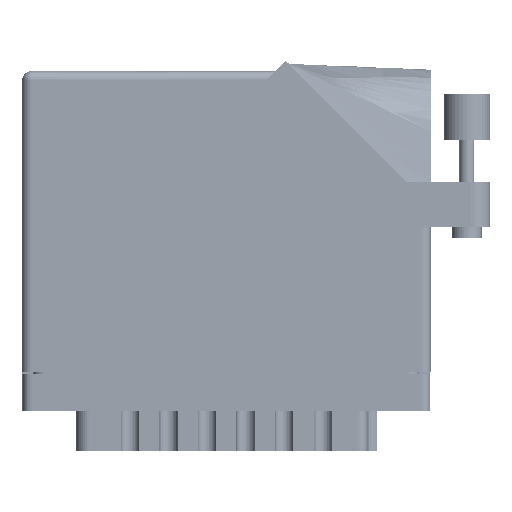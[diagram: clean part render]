
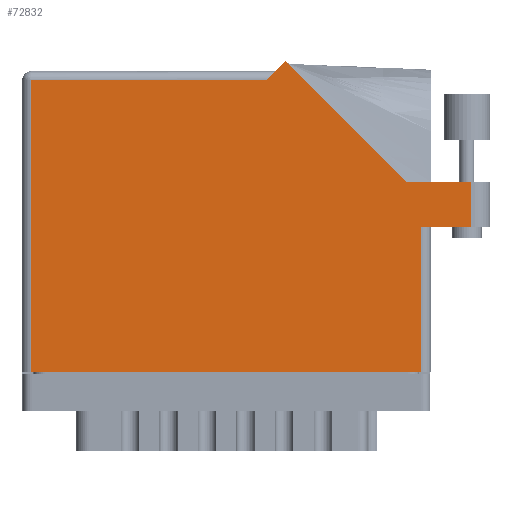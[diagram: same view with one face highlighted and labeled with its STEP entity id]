
A CAD part, front view. The second image highlights one B-rep face of the part: STEP entity #72832.
In plain terms, the highlighted face is planar.
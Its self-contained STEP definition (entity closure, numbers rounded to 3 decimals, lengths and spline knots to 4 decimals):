
#4905 = CARTESIAN_POINT ( 'NONE',  ( 0., 1.968, 0. ) ) ;
#5638 = CARTESIAN_POINT ( 'NONE',  ( 0., 2.03, 0. ) ) ;
#6931 = LINE ( 'NONE', #53528, #57470 ) ;
#7998 = EDGE_CURVE ( 'NONE', #71856, #78799, #75093, .T. ) ;
#9601 = VERTEX_POINT ( 'NONE', #84954 ) ;
#10204 = EDGE_CURVE ( 'NONE', #71552, #9601, #36644, .T. ) ;
#10798 = LINE ( 'NONE', #4905, #80476 ) ;
#12961 = CARTESIAN_POINT ( 'NONE',  ( 1.643, 1.968, 0. ) ) ;
#13494 = EDGE_LOOP ( 'NONE', ( #43923, #25591, #16066, #30915, #53617, #55203, #21313, #58799, #81192 ) ) ;
#13586 = CARTESIAN_POINT ( 'NONE',  ( 0., 0., 0. ) ) ;
#13745 = CARTESIAN_POINT ( 'NONE',  ( 3.155, 1.287, 0. ) ) ;
#14308 = DIRECTION ( 'NONE',  ( 1., 0., 0. ) ) ;
#14801 = VERTEX_POINT ( 'NONE', #86908 ) ;
#16066 = ORIENTED_EDGE ( 'NONE', *, *, #7998, .T. ) ;
#16969 = VECTOR ( 'NONE', #73017, 39.3701 ) ;
#19420 = DIRECTION ( 'NONE',  ( 0., 0., -1. ) ) ;
#21313 = ORIENTED_EDGE ( 'NONE', *, *, #48094, .T. ) ;
#22695 = DIRECTION ( 'NONE',  ( 1., 0., 0. ) ) ;
#22903 = DIRECTION ( 'NONE',  ( 0., 1., 0. ) ) ;
#23360 = CARTESIAN_POINT ( 'NONE',  ( 3.03, 1.287, 0. ) ) ;
#24436 = CARTESIAN_POINT ( 'NONE',  ( 0.062, 0., 0. ) ) ;
#25302 = VERTEX_POINT ( 'NONE', #70182 ) ;
#25591 = ORIENTED_EDGE ( 'NONE', *, *, #79175, .T. ) ;
#26758 = VECTOR ( 'NONE', #59239, 39.3701 ) ;
#30915 = ORIENTED_EDGE ( 'NONE', *, *, #80389, .T. ) ;
#31185 = DIRECTION ( 'NONE',  ( -0.707, 0.707, 0. ) ) ;
#34341 = VECTOR ( 'NONE', #22695, 39.3701 ) ;
#36644 = LINE ( 'NONE', #13586, #34341 ) ;
#38590 = DIRECTION ( 'NONE',  ( 0., -1., 0. ) ) ;
#43007 = VERTEX_POINT ( 'NONE', #84961 ) ;
#43923 = ORIENTED_EDGE ( 'NONE', *, *, #56450, .T. ) ;
#46718 = EDGE_CURVE ( 'NONE', #14801, #53883, #68690, .T. ) ;
#47881 = DIRECTION ( 'NONE',  ( -1., 0., 0. ) ) ;
#48024 = PLANE ( 'NONE',  #80949 ) ;
#48094 = EDGE_CURVE ( 'NONE', #43007, #71552, #80827, .T. ) ;
#49287 = VECTOR ( 'NONE', #72894, 39.3701 ) ;
#49854 = LINE ( 'NONE', #72097, #84590 ) ;
#50778 = VERTEX_POINT ( 'NONE', #72921 ) ;
#53528 = CARTESIAN_POINT ( 'NONE',  ( 2.5894, 1.287, 0. ) ) ;
#53617 = ORIENTED_EDGE ( 'NONE', *, *, #46718, .T. ) ;
#53883 = VERTEX_POINT ( 'NONE', #12961 ) ;
#55203 = ORIENTED_EDGE ( 'NONE', *, *, #65102, .T. ) ;
#56450 = EDGE_CURVE ( 'NONE', #25302, #50778, #49854, .T. ) ;
#57470 = VECTOR ( 'NONE', #31185, 39.3701 ) ;
#58799 = ORIENTED_EDGE ( 'NONE', *, *, #10204, .T. ) ;
#59239 = DIRECTION ( 'NONE',  ( -1., 0., 0. ) ) ;
#61602 = LINE ( 'NONE', #86400, #49287 ) ;
#62730 = DIRECTION ( 'NONE',  ( -1., 0., 0. ) ) ;
#65099 = CARTESIAN_POINT ( 'NONE',  ( 0.062, 0., 0. ) ) ;
#65102 = EDGE_CURVE ( 'NONE', #53883, #43007, #10798, .T. ) ;
#68690 = LINE ( 'NONE', #72099, #16969 ) ;
#70182 = CARTESIAN_POINT ( 'NONE',  ( 2.693, 0.98, 0. ) ) ;
#71552 = VERTEX_POINT ( 'NONE', #65099 ) ;
#71856 = VERTEX_POINT ( 'NONE', #23360 ) ;
#72097 = CARTESIAN_POINT ( 'NONE',  ( 2.755, 0.98, 0. ) ) ;
#72099 = CARTESIAN_POINT ( 'NONE',  ( 1.705, 2.03, 0. ) ) ;
#72832 = ADVANCED_FACE ( 'NONE', ( #77799 ), #48024, .F. ) ;
#72842 = LINE ( 'NONE', #80706, #89682 ) ;
#72894 = DIRECTION ( 'NONE',  ( 0., 1., 0. ) ) ;
#72921 = CARTESIAN_POINT ( 'NONE',  ( 3.03, 0.98, 0. ) ) ;
#73017 = DIRECTION ( 'NONE',  ( -0.707, -0.707, 0. ) ) ;
#75093 = LINE ( 'NONE', #13745, #26758 ) ;
#76972 = CARTESIAN_POINT ( 'NONE',  ( 2.5894, 1.287, 0. ) ) ;
#77799 = FACE_OUTER_BOUND ( 'NONE', #13494, .T. ) ;
#78799 = VERTEX_POINT ( 'NONE', #76972 ) ;
#79175 = EDGE_CURVE ( 'NONE', #50778, #71856, #72842, .T. ) ;
#80389 = EDGE_CURVE ( 'NONE', #78799, #14801, #6931, .T. ) ;
#80476 = VECTOR ( 'NONE', #47881, 39.3701 ) ;
#80706 = CARTESIAN_POINT ( 'NONE',  ( 3.03, 1.287, 0. ) ) ;
#80827 = LINE ( 'NONE', #24436, #84124 ) ;
#80949 = AXIS2_PLACEMENT_3D ( 'NONE', #5638, #19420, #62730 ) ;
#81192 = ORIENTED_EDGE ( 'NONE', *, *, #82716, .T. ) ;
#82716 = EDGE_CURVE ( 'NONE', #9601, #25302, #61602, .T. ) ;
#84124 = VECTOR ( 'NONE', #38590, 39.3701 ) ;
#84590 = VECTOR ( 'NONE', #14308, 39.3701 ) ;
#84954 = CARTESIAN_POINT ( 'NONE',  ( 2.693, 0., 0. ) ) ;
#84961 = CARTESIAN_POINT ( 'NONE',  ( 0.062, 1.968, 0. ) ) ;
#86400 = CARTESIAN_POINT ( 'NONE',  ( 2.693, 0.98, 0. ) ) ;
#86908 = CARTESIAN_POINT ( 'NONE',  ( 1.7757, 2.1007, 0. ) ) ;
#89682 = VECTOR ( 'NONE', #22903, 39.3701 ) ;
